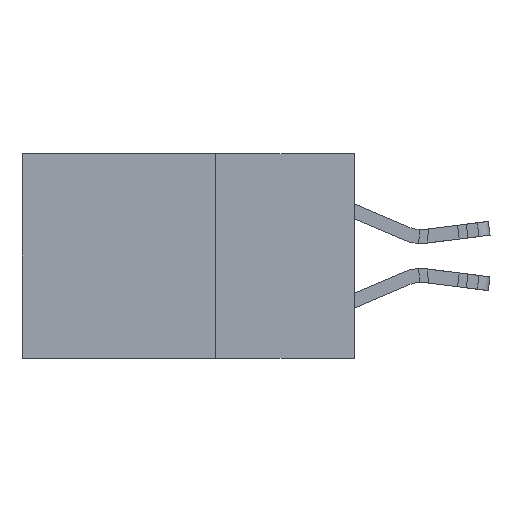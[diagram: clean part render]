
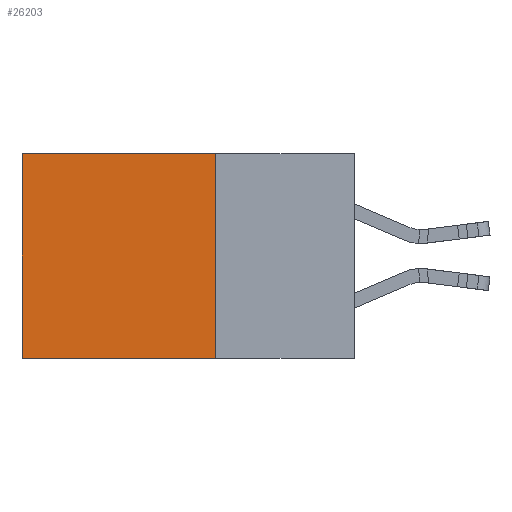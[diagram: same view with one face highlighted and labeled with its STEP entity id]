
A CAD part, left-side view. The second image highlights one B-rep face of the part: STEP entity #26203.
In plain terms, the highlighted planar face has unit normal (-1, 0, 0).
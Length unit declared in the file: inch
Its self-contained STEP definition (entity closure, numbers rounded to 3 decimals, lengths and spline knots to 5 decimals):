
#767 = VERTEX_POINT ( 'NONE', #1129 ) ;
#798 = AXIS2_PLACEMENT_3D ( 'NONE', #5073, #22808, #7637 ) ;
#1129 = CARTESIAN_POINT ( 'NONE',  ( 0.298, 0.6, -0.37 ) ) ;
#1630 = CARTESIAN_POINT ( 'NONE',  ( 0.298, 0.6, 0. ) ) ;
#2219 = LINE ( 'NONE', #23258, #14932 ) ;
#3864 = ORIENTED_EDGE ( 'NONE', *, *, #6660, .F. ) ;
#4370 = EDGE_CURVE ( 'NONE', #5693, #767, #18175, .T. ) ;
#5073 = CARTESIAN_POINT ( 'NONE',  ( 0.298, 0.25, 0. ) ) ;
#5492 = LINE ( 'NONE', #19106, #31716 ) ;
#5693 = VERTEX_POINT ( 'NONE', #11377 ) ;
#6018 = DIRECTION ( 'NONE',  ( 0., 1., 0. ) ) ;
#6161 = CARTESIAN_POINT ( 'NONE',  ( 0.298, 0.25, 0. ) ) ;
#6660 = EDGE_CURVE ( 'NONE', #29777, #5693, #31994, .T. ) ;
#7637 = DIRECTION ( 'NONE',  ( 0., 0., -1. ) ) ;
#9015 = DIRECTION ( 'NONE',  ( 0., 0., -1. ) ) ;
#9334 = VECTOR ( 'NONE', #18058, 39.37008 ) ;
#10636 = VECTOR ( 'NONE', #6018, 39.37008 ) ;
#11377 = CARTESIAN_POINT ( 'NONE',  ( 0.298, 0.25, -0.37 ) ) ;
#14932 = VECTOR ( 'NONE', #25853, 39.37008 ) ;
#15492 = CARTESIAN_POINT ( 'NONE',  ( 0.298, 0.25, 0. ) ) ;
#16851 = ORIENTED_EDGE ( 'NONE', *, *, #31273, .T. ) ;
#17559 = FACE_OUTER_BOUND ( 'NONE', #29809, .T. ) ;
#18058 = DIRECTION ( 'NONE',  ( 0., 0., -1. ) ) ;
#18175 = LINE ( 'NONE', #26357, #10636 ) ;
#19106 = CARTESIAN_POINT ( 'NONE',  ( 0.298, 0.6, 0. ) ) ;
#19261 = ORIENTED_EDGE ( 'NONE', *, *, #4370, .F. ) ;
#22808 = DIRECTION ( 'NONE',  ( 1., 0., 0. ) ) ;
#23258 = CARTESIAN_POINT ( 'NONE',  ( 0.298, 0.25, 0. ) ) ;
#25435 = ORIENTED_EDGE ( 'NONE', *, *, #32265, .T. ) ;
#25853 = DIRECTION ( 'NONE',  ( 0., 1., 0. ) ) ;
#26203 = ADVANCED_FACE ( 'NONE', ( #17559 ), #30423, .F. ) ;
#26357 = CARTESIAN_POINT ( 'NONE',  ( 0.298, 0.25, -0.37 ) ) ;
#29777 = VERTEX_POINT ( 'NONE', #6161 ) ;
#29809 = EDGE_LOOP ( 'NONE', ( #16851, #19261, #3864, #25435 ) ) ;
#30423 = PLANE ( 'NONE',  #798 ) ;
#31273 = EDGE_CURVE ( 'NONE', #31923, #767, #5492, .T. ) ;
#31716 = VECTOR ( 'NONE', #9015, 39.37008 ) ;
#31923 = VERTEX_POINT ( 'NONE', #1630 ) ;
#31994 = LINE ( 'NONE', #15492, #9334 ) ;
#32265 = EDGE_CURVE ( 'NONE', #29777, #31923, #2219, .T. ) ;
